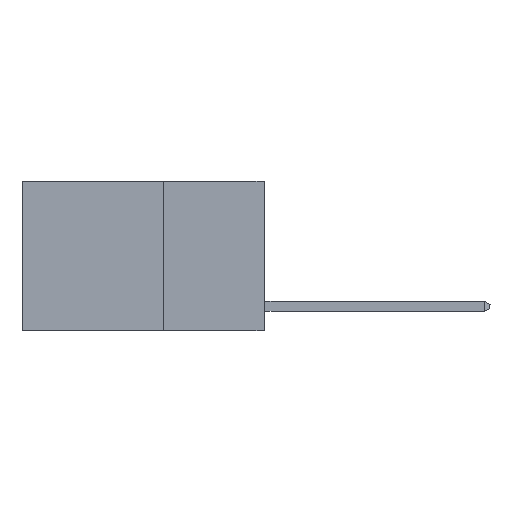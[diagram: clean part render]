
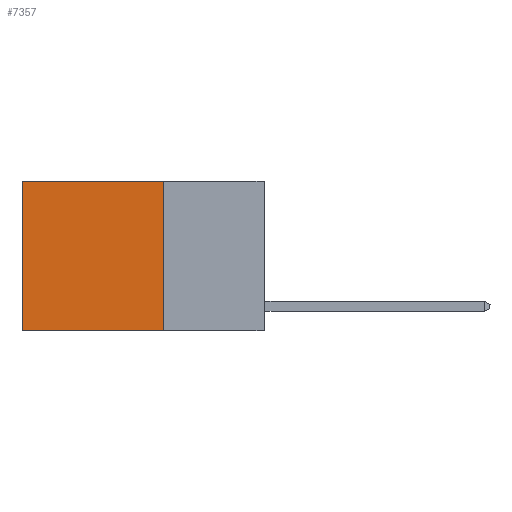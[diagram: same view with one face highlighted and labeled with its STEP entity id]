
A CAD part, left-side view. The second image highlights one B-rep face of the part: STEP entity #7357.
In plain terms, the highlighted planar face has unit normal (-1, 0, 0).
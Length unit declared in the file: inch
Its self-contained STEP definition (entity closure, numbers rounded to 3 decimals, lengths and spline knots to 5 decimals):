
#502 = CARTESIAN_POINT ( 'NONE',  ( 0.2625, 0.6, -0.37 ) ) ;
#580 = EDGE_CURVE ( 'NONE', #2745, #2026, #4210, .T. ) ;
#742 = ORIENTED_EDGE ( 'NONE', *, *, #6897, .T. ) ;
#842 = DIRECTION ( 'NONE',  ( 1., 0., 0. ) ) ;
#1545 = DIRECTION ( 'NONE',  ( 0., 0., -1. ) ) ;
#1641 = DIRECTION ( 'NONE',  ( 0., 0., -1. ) ) ;
#1995 = VECTOR ( 'NONE', #2801, 39.37008 ) ;
#2026 = VERTEX_POINT ( 'NONE', #4309 ) ;
#2094 = EDGE_LOOP ( 'NONE', ( #5767, #4258, #3009, #742 ) ) ;
#2310 = PLANE ( 'NONE',  #5737 ) ;
#2705 = VECTOR ( 'NONE', #3436, 39.37008 ) ;
#2745 = VERTEX_POINT ( 'NONE', #4096 ) ;
#2765 = VERTEX_POINT ( 'NONE', #4961 ) ;
#2801 = DIRECTION ( 'NONE',  ( 0., 0., -1. ) ) ;
#2902 = EDGE_CURVE ( 'NONE', #2026, #4616, #8856, .T. ) ;
#3009 = ORIENTED_EDGE ( 'NONE', *, *, #580, .F. ) ;
#3199 = VECTOR ( 'NONE', #1545, 39.37008 ) ;
#3436 = DIRECTION ( 'NONE',  ( 0., 1., 0. ) ) ;
#4096 = CARTESIAN_POINT ( 'NONE',  ( 0.2625, 0.25, 0. ) ) ;
#4188 = EDGE_CURVE ( 'NONE', #2765, #4616, #5995, .T. ) ;
#4210 = LINE ( 'NONE', #4330, #1995 ) ;
#4258 = ORIENTED_EDGE ( 'NONE', *, *, #2902, .F. ) ;
#4309 = CARTESIAN_POINT ( 'NONE',  ( 0.2625, 0.25, -0.37 ) ) ;
#4315 = CARTESIAN_POINT ( 'NONE',  ( 0.2625, 0.25, -0.37 ) ) ;
#4330 = CARTESIAN_POINT ( 'NONE',  ( 0.2625, 0.25, 0. ) ) ;
#4616 = VERTEX_POINT ( 'NONE', #502 ) ;
#4961 = CARTESIAN_POINT ( 'NONE',  ( 0.2625, 0.6, 0. ) ) ;
#5200 = FACE_OUTER_BOUND ( 'NONE', #2094, .T. ) ;
#5383 = DIRECTION ( 'NONE',  ( 0., 1., 0. ) ) ;
#5737 = AXIS2_PLACEMENT_3D ( 'NONE', #8562, #842, #1641 ) ;
#5767 = ORIENTED_EDGE ( 'NONE', *, *, #4188, .T. ) ;
#5995 = LINE ( 'NONE', #6278, #3199 ) ;
#6278 = CARTESIAN_POINT ( 'NONE',  ( 0.2625, 0.6, 0. ) ) ;
#6313 = LINE ( 'NONE', #10002, #7625 ) ;
#6897 = EDGE_CURVE ( 'NONE', #2745, #2765, #6313, .T. ) ;
#7357 = ADVANCED_FACE ( 'NONE', ( #5200 ), #2310, .F. ) ;
#7625 = VECTOR ( 'NONE', #5383, 39.37008 ) ;
#8562 = CARTESIAN_POINT ( 'NONE',  ( 0.2625, 0.25, 0. ) ) ;
#8856 = LINE ( 'NONE', #4315, #2705 ) ;
#10002 = CARTESIAN_POINT ( 'NONE',  ( 0.2625, 0.25, 0. ) ) ;
